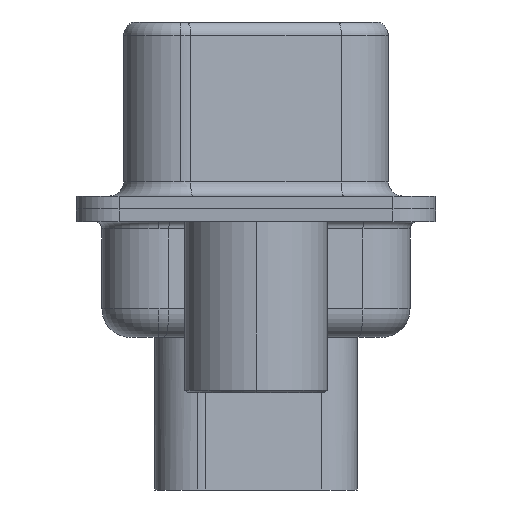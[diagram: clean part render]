
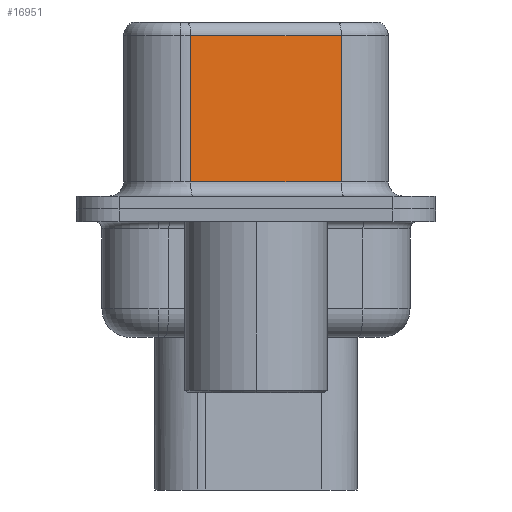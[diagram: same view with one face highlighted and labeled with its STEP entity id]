
A CAD part, left-side view. The second image highlights one B-rep face of the part: STEP entity #16951.
In plain terms, the highlighted planar face has unit normal (-0.985, -0.174, 0).
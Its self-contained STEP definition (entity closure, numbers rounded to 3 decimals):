
#439 = EDGE_CURVE ( 'NONE', #7915, #4924, #16300, .T. ) ;
#444 = EDGE_CURVE ( 'NONE', #7915, #10661, #6795, .T. ) ;
#1569 = ORIENTED_EDGE ( 'NONE', *, *, #444, .T. ) ;
#3049 = VECTOR ( 'NONE', #5268, 1000. ) ;
#4162 = VECTOR ( 'NONE', #13967, 1000. ) ;
#4279 = EDGE_CURVE ( 'NONE', #14511, #4924, #17014, .T. ) ;
#4924 = VERTEX_POINT ( 'NONE', #10390 ) ;
#5268 = DIRECTION ( 'NONE',  ( 0., 0., -1. ) ) ;
#5522 = CARTESIAN_POINT ( 'NONE',  ( 4.551, -2.987, 6.57 ) ) ;
#6196 = DIRECTION ( 'NONE',  ( 0.174, -0.985, 0. ) ) ;
#6795 = LINE ( 'NONE', #15848, #4162 ) ;
#7011 = CARTESIAN_POINT ( 'NONE',  ( 3.62, 2.293, 6.57 ) ) ;
#7732 = EDGE_CURVE ( 'NONE', #10661, #14511, #10550, .T. ) ;
#7915 = VERTEX_POINT ( 'NONE', #19101 ) ;
#8664 = CARTESIAN_POINT ( 'NONE',  ( 4.551, -2.987, 6.57 ) ) ;
#10064 = CARTESIAN_POINT ( 'NONE',  ( 4.551, -2.987, 0.95 ) ) ;
#10132 = ORIENTED_EDGE ( 'NONE', *, *, #4279, .T. ) ;
#10350 = EDGE_LOOP ( 'NONE', ( #16286, #1569, #17464, #10132 ) ) ;
#10390 = CARTESIAN_POINT ( 'NONE',  ( 4.551, -2.987, 0.95 ) ) ;
#10550 = LINE ( 'NONE', #7011, #10838 ) ;
#10661 = VERTEX_POINT ( 'NONE', #20034 ) ;
#10686 = FACE_OUTER_BOUND ( 'NONE', #10350, .T. ) ;
#10718 = AXIS2_PLACEMENT_3D ( 'NONE', #5522, #17523, #19397 ) ;
#10838 = VECTOR ( 'NONE', #21360, 1000. ) ;
#13967 = DIRECTION ( 'NONE',  ( -0.174, 0.985, 0. ) ) ;
#14511 = VERTEX_POINT ( 'NONE', #16758 ) ;
#15848 = CARTESIAN_POINT ( 'NONE',  ( 4.551, -2.987, 6.07 ) ) ;
#16286 = ORIENTED_EDGE ( 'NONE', *, *, #439, .F. ) ;
#16300 = LINE ( 'NONE', #8664, #3049 ) ;
#16758 = CARTESIAN_POINT ( 'NONE',  ( 3.62, 2.293, 0.95 ) ) ;
#16951 = ADVANCED_FACE ( 'NONE', ( #10686 ), #17874, .F. ) ;
#17014 = LINE ( 'NONE', #10064, #19102 ) ;
#17464 = ORIENTED_EDGE ( 'NONE', *, *, #7732, .T. ) ;
#17523 = DIRECTION ( 'NONE',  ( 0.985, 0.174, 0. ) ) ;
#17874 = PLANE ( 'NONE',  #10718 ) ;
#19101 = CARTESIAN_POINT ( 'NONE',  ( 4.551, -2.987, 6.07 ) ) ;
#19102 = VECTOR ( 'NONE', #6196, 1000. ) ;
#19397 = DIRECTION ( 'NONE',  ( -0.174, 0.985, 0. ) ) ;
#20034 = CARTESIAN_POINT ( 'NONE',  ( 3.62, 2.293, 6.07 ) ) ;
#21360 = DIRECTION ( 'NONE',  ( 0., 0., -1. ) ) ;
